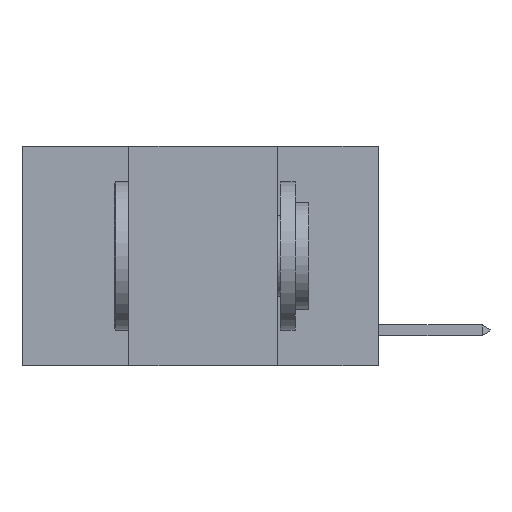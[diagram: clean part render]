
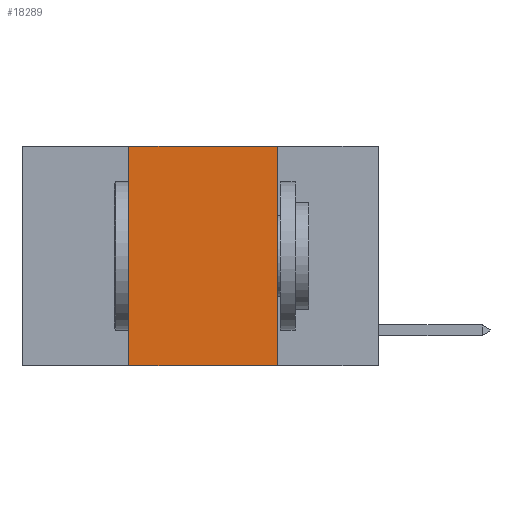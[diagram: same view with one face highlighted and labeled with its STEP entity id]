
A CAD part, left-side view. The second image highlights one B-rep face of the part: STEP entity #18289.
In plain terms, the highlighted planar face has unit normal (-1, 0, 0).
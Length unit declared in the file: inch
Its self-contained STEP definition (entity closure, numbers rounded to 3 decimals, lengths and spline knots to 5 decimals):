
#1115 = FACE_OUTER_BOUND ( 'NONE', #11011, .T. ) ;
#1263 = CARTESIAN_POINT ( 'NONE',  ( 0., 0.17, 0. ) ) ;
#1790 = CARTESIAN_POINT ( 'NONE',  ( 0., 0.42, 0. ) ) ;
#2662 = VECTOR ( 'NONE', #19791, 39.37008 ) ;
#3132 = CARTESIAN_POINT ( 'NONE',  ( 0., 0.17, -0.37 ) ) ;
#3369 = LINE ( 'NONE', #11558, #15651 ) ;
#3975 = AXIS2_PLACEMENT_3D ( 'NONE', #7787, #19764, #11487 ) ;
#4499 = PLANE ( 'NONE',  #3975 ) ;
#4843 = CARTESIAN_POINT ( 'NONE',  ( 0., 0.6, 0. ) ) ;
#5388 = LINE ( 'NONE', #1790, #8843 ) ;
#7520 = VERTEX_POINT ( 'NONE', #12880 ) ;
#7787 = CARTESIAN_POINT ( 'NONE',  ( 0., 0.6, 0. ) ) ;
#8262 = CARTESIAN_POINT ( 'NONE',  ( 0., 0.17, 0. ) ) ;
#8330 = CARTESIAN_POINT ( 'NONE',  ( 0., 0.42, 0. ) ) ;
#8843 = VECTOR ( 'NONE', #15446, 39.37008 ) ;
#9319 = ORIENTED_EDGE ( 'NONE', *, *, #20908, .F. ) ;
#9952 = VERTEX_POINT ( 'NONE', #8330 ) ;
#11011 = EDGE_LOOP ( 'NONE', ( #13805, #9319, #14818, #15099 ) ) ;
#11418 = EDGE_CURVE ( 'NONE', #7520, #16313, #3369, .T. ) ;
#11487 = DIRECTION ( 'NONE',  ( 0., 0., -1. ) ) ;
#11558 = CARTESIAN_POINT ( 'NONE',  ( 0., 0.6, -0.37 ) ) ;
#12623 = LINE ( 'NONE', #1263, #16772 ) ;
#12880 = CARTESIAN_POINT ( 'NONE',  ( 0., 0.42, -0.37 ) ) ;
#13119 = EDGE_CURVE ( 'NONE', #13649, #16313, #12623, .T. ) ;
#13649 = VERTEX_POINT ( 'NONE', #8262 ) ;
#13805 = ORIENTED_EDGE ( 'NONE', *, *, #13119, .F. ) ;
#14818 = ORIENTED_EDGE ( 'NONE', *, *, #18035, .F. ) ;
#15099 = ORIENTED_EDGE ( 'NONE', *, *, #11418, .T. ) ;
#15446 = DIRECTION ( 'NONE',  ( 0., 0., 1. ) ) ;
#15651 = VECTOR ( 'NONE', #21377, 39.37008 ) ;
#16313 = VERTEX_POINT ( 'NONE', #3132 ) ;
#16772 = VECTOR ( 'NONE', #19280, 39.37008 ) ;
#18035 = EDGE_CURVE ( 'NONE', #7520, #9952, #5388, .T. ) ;
#18278 = LINE ( 'NONE', #4843, #2662 ) ;
#18289 = ADVANCED_FACE ( 'NONE', ( #1115 ), #4499, .F. ) ;
#19280 = DIRECTION ( 'NONE',  ( 0., 0., -1. ) ) ;
#19764 = DIRECTION ( 'NONE',  ( 1., 0., 0. ) ) ;
#19791 = DIRECTION ( 'NONE',  ( 0., -1., 0. ) ) ;
#20908 = EDGE_CURVE ( 'NONE', #9952, #13649, #18278, .T. ) ;
#21377 = DIRECTION ( 'NONE',  ( 0., -1., 0. ) ) ;
